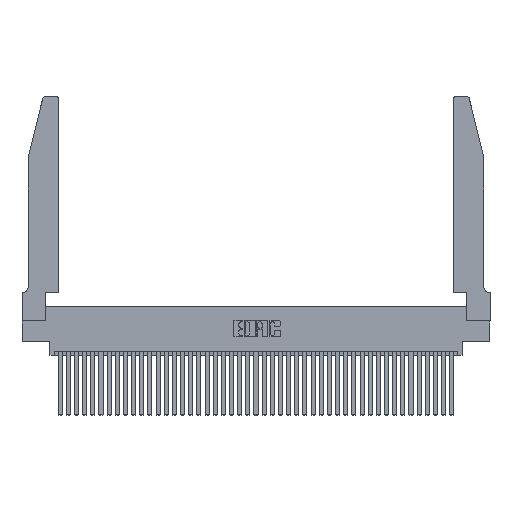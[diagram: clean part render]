
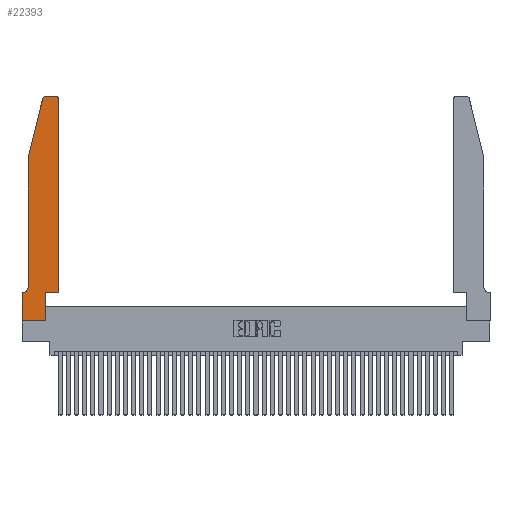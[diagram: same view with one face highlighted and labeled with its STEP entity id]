
A CAD part, top view. The second image highlights one B-rep face of the part: STEP entity #22393.
In plain terms, the highlighted planar face has unit normal (0, 0, 1).
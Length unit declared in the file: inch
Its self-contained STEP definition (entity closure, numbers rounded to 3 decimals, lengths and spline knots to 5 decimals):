
#131 = DIRECTION ( 'NONE',  ( 1., 0., 0. ) ) ;
#859 = VERTEX_POINT ( 'NONE', #15776 ) ;
#909 = ORIENTED_EDGE ( 'NONE', *, *, #8265, .T. ) ;
#1089 = VERTEX_POINT ( 'NONE', #39410 ) ;
#1284 = CARTESIAN_POINT ( 'NONE',  ( 0.0755, 2., 0.37 ) ) ;
#1513 = ORIENTED_EDGE ( 'NONE', *, *, #20522, .T. ) ;
#1703 = ORIENTED_EDGE ( 'NONE', *, *, #24826, .T. ) ;
#1908 = LINE ( 'NONE', #26168, #18284 ) ;
#1973 = LINE ( 'NONE', #6899, #9641 ) ;
#3145 = CARTESIAN_POINT ( 'NONE',  ( 0.284, 2.75, 0.37 ) ) ;
#3201 = VERTEX_POINT ( 'NONE', #15417 ) ;
#3535 = VECTOR ( 'NONE', #20845, 39.37008 ) ;
#3860 = ORIENTED_EDGE ( 'NONE', *, *, #16978, .T. ) ;
#4255 = ORIENTED_EDGE ( 'NONE', *, *, #19692, .T. ) ;
#4336 = CARTESIAN_POINT ( 'NONE',  ( 0.4505, 2.72, 0.37 ) ) ;
#4340 = VERTEX_POINT ( 'NONE', #24080 ) ;
#4625 = AXIS2_PLACEMENT_3D ( 'NONE', #16420, #19732, #131 ) ;
#4912 = CIRCLE ( 'NONE', #41874, 0.03 ) ;
#6559 = AXIS2_PLACEMENT_3D ( 'NONE', #7854, #30766, #11170 ) ;
#6898 = FACE_OUTER_BOUND ( 'NONE', #21249, .T. ) ;
#6899 = CARTESIAN_POINT ( 'NONE',  ( 0.0755, 0.35, 0.37 ) ) ;
#7838 = CARTESIAN_POINT ( 'NONE',  ( 0., 0., 0.37 ) ) ;
#7854 = CARTESIAN_POINT ( 'NONE',  ( 0.0055, 0.42, 0.37 ) ) ;
#8265 = EDGE_CURVE ( 'NONE', #1089, #3201, #12190, .T. ) ;
#8653 = VERTEX_POINT ( 'NONE', #3145 ) ;
#9288 = EDGE_CURVE ( 'NONE', #8653, #859, #17736, .T. ) ;
#9523 = DIRECTION ( 'NONE',  ( 0., 0., 1. ) ) ;
#9641 = VECTOR ( 'NONE', #26547, 39.37008 ) ;
#9962 = DIRECTION ( 'NONE',  ( 0., 0., 1. ) ) ;
#10062 = EDGE_CURVE ( 'NONE', #4340, #38080, #17149, .T. ) ;
#11170 = DIRECTION ( 'NONE',  ( -1., 0., 0. ) ) ;
#11499 = CARTESIAN_POINT ( 'NONE',  ( 0., 0., 0.37 ) ) ;
#12190 = CIRCLE ( 'NONE', #6559, 0.07 ) ;
#12229 = LINE ( 'NONE', #33771, #3535 ) ;
#12542 = ORIENTED_EDGE ( 'NONE', *, *, #25617, .T. ) ;
#13327 = DIRECTION ( 'NONE',  ( 0., 1., 0. ) ) ;
#13612 = ORIENTED_EDGE ( 'NONE', *, *, #28708, .T. ) ;
#13898 = VERTEX_POINT ( 'NONE', #41176 ) ;
#15268 = DIRECTION ( 'NONE',  ( 0., -1., 0. ) ) ;
#15417 = CARTESIAN_POINT ( 'NONE',  ( 0.0055, 0.35, 0.37 ) ) ;
#15776 = CARTESIAN_POINT ( 'NONE',  ( 0.25487, 2.72718, 0.37 ) ) ;
#16420 = CARTESIAN_POINT ( 'NONE',  ( 0., 0.35, 0.37 ) ) ;
#16978 = EDGE_CURVE ( 'NONE', #18656, #1089, #19103, .T. ) ;
#17149 = LINE ( 'NONE', #29650, #41111 ) ;
#17272 = AXIS2_PLACEMENT_3D ( 'NONE', #29126, #9523, #32380 ) ;
#17647 = VERTEX_POINT ( 'NONE', #11499 ) ;
#17736 = CIRCLE ( 'NONE', #17272, 0.03 ) ;
#17752 = DIRECTION ( 'NONE',  ( 1., 0., 0. ) ) ;
#18284 = VECTOR ( 'NONE', #35950, 39.37008 ) ;
#18656 = VERTEX_POINT ( 'NONE', #1284 ) ;
#19103 = LINE ( 'NONE', #34813, #36421 ) ;
#19217 = CARTESIAN_POINT ( 'NONE',  ( 0.2605, 2.75, 0.37 ) ) ;
#19264 = EDGE_CURVE ( 'NONE', #13898, #28954, #12229, .T. ) ;
#19692 = EDGE_CURVE ( 'NONE', #36988, #8653, #40254, .T. ) ;
#19732 = DIRECTION ( 'NONE',  ( 0., 0., 1. ) ) ;
#20522 = EDGE_CURVE ( 'NONE', #40532, #17647, #1908, .T. ) ;
#20845 = DIRECTION ( 'NONE',  ( 0., 1., 0. ) ) ;
#21129 = ORIENTED_EDGE ( 'NONE', *, *, #24317, .T. ) ;
#21249 = EDGE_LOOP ( 'NONE', ( #4255, #33248, #1703, #3860, #909, #21129, #1513, #13612, #41809, #29962, #22820, #12542 ) ) ;
#22393 = ADVANCED_FACE ( 'NONE', ( #6898 ), #35955, .T. ) ;
#22820 = ORIENTED_EDGE ( 'NONE', *, *, #10062, .T. ) ;
#24080 = CARTESIAN_POINT ( 'NONE',  ( 0.4505, 0.35, 0.37 ) ) ;
#24317 = EDGE_CURVE ( 'NONE', #3201, #40532, #1973, .T. ) ;
#24706 = LINE ( 'NONE', #7838, #39931 ) ;
#24826 = EDGE_CURVE ( 'NONE', #859, #18656, #24984, .T. ) ;
#24984 = LINE ( 'NONE', #42221, #40193 ) ;
#25617 = EDGE_CURVE ( 'NONE', #38080, #36988, #4912, .T. ) ;
#25826 = DIRECTION ( 'NONE',  ( 1., 0., 0. ) ) ;
#26064 = DIRECTION ( 'NONE',  ( -0.239, -0.971, 0. ) ) ;
#26168 = CARTESIAN_POINT ( 'NONE',  ( 0., 0., 0.37 ) ) ;
#26547 = DIRECTION ( 'NONE',  ( -1., 0., 0. ) ) ;
#26818 = CARTESIAN_POINT ( 'NONE',  ( 0., 0.35, 0.37 ) ) ;
#28708 = EDGE_CURVE ( 'NONE', #17647, #13898, #24706, .T. ) ;
#28954 = VERTEX_POINT ( 'NONE', #31872 ) ;
#29126 = CARTESIAN_POINT ( 'NONE',  ( 0.284, 2.72, 0.37 ) ) ;
#29577 = CARTESIAN_POINT ( 'NONE',  ( 0.4205, 2.72, 0.37 ) ) ;
#29650 = CARTESIAN_POINT ( 'NONE',  ( 0.4505, 0.35, 0.37 ) ) ;
#29962 = ORIENTED_EDGE ( 'NONE', *, *, #33123, .T. ) ;
#30766 = DIRECTION ( 'NONE',  ( 0., 0., -1. ) ) ;
#31872 = CARTESIAN_POINT ( 'NONE',  ( 0.2865, 0.35, 0.37 ) ) ;
#32213 = CARTESIAN_POINT ( 'NONE',  ( 0.4505, 0.35, 0.37 ) ) ;
#32380 = DIRECTION ( 'NONE',  ( 1., 0., 0. ) ) ;
#32452 = VECTOR ( 'NONE', #25826, 39.37008 ) ;
#32834 = DIRECTION ( 'NONE',  ( 1., 0., 0. ) ) ;
#33123 = EDGE_CURVE ( 'NONE', #28954, #4340, #41081, .T. ) ;
#33248 = ORIENTED_EDGE ( 'NONE', *, *, #9288, .T. ) ;
#33771 = CARTESIAN_POINT ( 'NONE',  ( 0.2865, 0.35, 0.37 ) ) ;
#34813 = CARTESIAN_POINT ( 'NONE',  ( 0.0755, 2., 0.37 ) ) ;
#35950 = DIRECTION ( 'NONE',  ( 0., -1., 0. ) ) ;
#35955 = PLANE ( 'NONE',  #4625 ) ;
#36235 = CARTESIAN_POINT ( 'NONE',  ( 0.4205, 2.75, 0.37 ) ) ;
#36421 = VECTOR ( 'NONE', #15268, 39.37008 ) ;
#36988 = VERTEX_POINT ( 'NONE', #36235 ) ;
#38080 = VERTEX_POINT ( 'NONE', #4336 ) ;
#39230 = VECTOR ( 'NONE', #41967, 39.37008 ) ;
#39410 = CARTESIAN_POINT ( 'NONE',  ( 0.0755, 0.42, 0.37 ) ) ;
#39931 = VECTOR ( 'NONE', #17752, 39.37008 ) ;
#40193 = VECTOR ( 'NONE', #26064, 39.37008 ) ;
#40254 = LINE ( 'NONE', #19217, #39230 ) ;
#40532 = VERTEX_POINT ( 'NONE', #26818 ) ;
#41081 = LINE ( 'NONE', #32213, #32452 ) ;
#41111 = VECTOR ( 'NONE', #13327, 39.37008 ) ;
#41176 = CARTESIAN_POINT ( 'NONE',  ( 0.2865, 0., 0.37 ) ) ;
#41809 = ORIENTED_EDGE ( 'NONE', *, *, #19264, .T. ) ;
#41874 = AXIS2_PLACEMENT_3D ( 'NONE', #29577, #9962, #32834 ) ;
#41967 = DIRECTION ( 'NONE',  ( -1., 0., 0. ) ) ;
#42221 = CARTESIAN_POINT ( 'NONE',  ( 0.0755, 2., 0.37 ) ) ;
